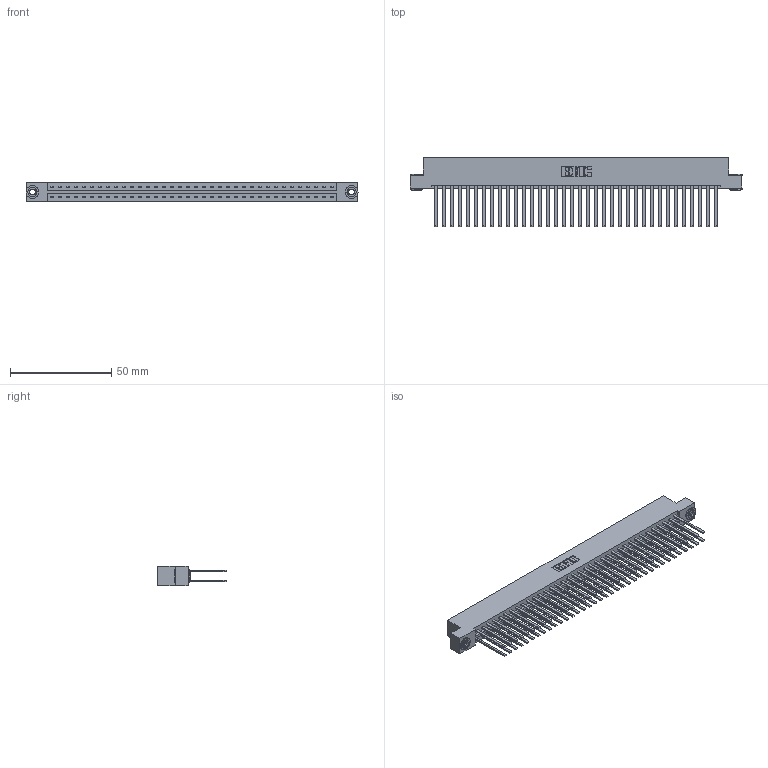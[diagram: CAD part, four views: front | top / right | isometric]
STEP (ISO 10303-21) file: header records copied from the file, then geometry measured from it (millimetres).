
FILE_DESCRIPTION (( 'STEP AP203' ), '1' );
FILE_NAME ('333-072-544-203.STEP', '2018-08-04T20:58:12', ( '' ), ( '' ), 'SwSTEP 2.0', 'SolidWorks 2016', '' );
FILE_SCHEMA (( 'CONFIG_CONTROL_DESIGN' ));
Length unit declared in the file: inch
Products named in the file (4): 333 Part_Flush - .156 Dia - TH; 345-292-001_345-293-144; 345-250-002_345-250-002-102; 333-072-544-203
Assembly tree (75 placements, depth 2):
  333-072-544-203
    333 Part_Flush - .156 Dia - TH
    345-292-001_345-293-144  x72
    345-250-002_345-250-002-102  x2
Bounding box: 164.19 x 34.3 x 9.4 mm (x, y, z)
Volume: 17735 mm3; surface area: 24373.3 mm2
Topology: 75 solids, 75 shells, 3464 faces, 10251 edges, 6734 vertices
Faces by surface type: plane 2384, cylinder 1072, cone 8
Entity records: 24402 total; most frequent: CARTESIAN_POINT 4025, ORIENTED_EDGE 3954, DIRECTION 3479, EDGE_CURVE 1977, VECTOR 1829, LINE 1829, VERTEX_POINT 1314, AXIS2_PLACEMENT_3D 825
